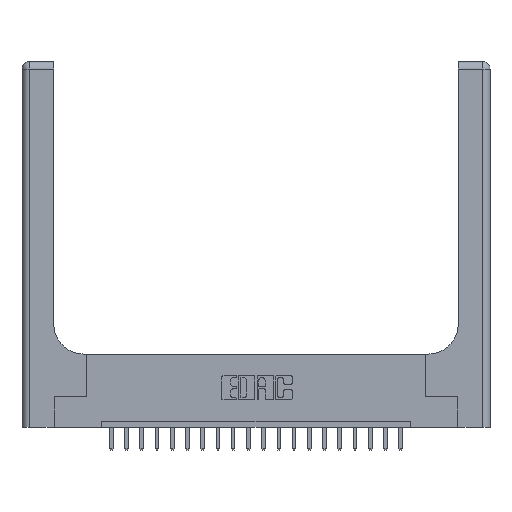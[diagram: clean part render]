
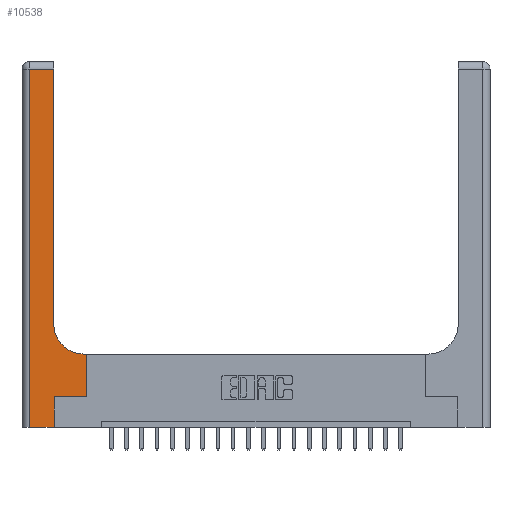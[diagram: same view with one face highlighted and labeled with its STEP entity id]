
A CAD part, top view. The second image highlights one B-rep face of the part: STEP entity #10538.
In plain terms, the highlighted planar face has unit normal (0, 0, 1).
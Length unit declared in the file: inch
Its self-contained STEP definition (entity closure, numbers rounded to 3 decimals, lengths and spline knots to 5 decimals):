
#203 = DIRECTION ( 'NONE',  ( 0., -1., 0. ) ) ;
#1177 = DIRECTION ( 'NONE',  ( 1., 0., 0. ) ) ;
#1221 = VECTOR ( 'NONE', #18222, 39.37008 ) ;
#1349 = CARTESIAN_POINT ( 'NONE',  ( 0.265, 0.25, 0.37 ) ) ;
#1490 = DIRECTION ( 'NONE',  ( 0., 1., 0. ) ) ;
#1596 = DIRECTION ( 'NONE',  ( 0., 0., -1. ) ) ;
#1726 = VECTOR ( 'NONE', #203, 39.37008 ) ;
#2391 = EDGE_CURVE ( 'NONE', #17876, #12855, #10352, .T. ) ;
#2981 = CARTESIAN_POINT ( 'NONE',  ( 0.51, 0.85, 0.37 ) ) ;
#3082 = ORIENTED_EDGE ( 'NONE', *, *, #6459, .T. ) ;
#4168 = LINE ( 'NONE', #12697, #9142 ) ;
#4330 = CARTESIAN_POINT ( 'NONE',  ( 0.26, 0.85, 0.37 ) ) ;
#4961 = ORIENTED_EDGE ( 'NONE', *, *, #12936, .T. ) ;
#4981 = ORIENTED_EDGE ( 'NONE', *, *, #11294, .T. ) ;
#5397 = EDGE_CURVE ( 'NONE', #9587, #10948, #16227, .T. ) ;
#5666 = AXIS2_PLACEMENT_3D ( 'NONE', #2981, #1596, #11240 ) ;
#5792 = VECTOR ( 'NONE', #6919, 39.37008 ) ;
#6413 = VERTEX_POINT ( 'NONE', #15447 ) ;
#6459 = EDGE_CURVE ( 'NONE', #13026, #11621, #8412, .T. ) ;
#6919 = DIRECTION ( 'NONE',  ( -1., 0., 0. ) ) ;
#7053 = DIRECTION ( 'NONE',  ( 1., 0., 0. ) ) ;
#7265 = EDGE_CURVE ( 'NONE', #11621, #8614, #4168, .T. ) ;
#7586 = VERTEX_POINT ( 'NONE', #11899 ) ;
#7779 = CARTESIAN_POINT ( 'NONE',  ( 0.06, 2.94, 0.37 ) ) ;
#8412 = LINE ( 'NONE', #17156, #13723 ) ;
#8614 = VERTEX_POINT ( 'NONE', #20523 ) ;
#8713 = LINE ( 'NONE', #10435, #1221 ) ;
#8873 = CARTESIAN_POINT ( 'NONE',  ( 0., 3., 0.37 ) ) ;
#8948 = DIRECTION ( 'NONE',  ( -1., 0., 0. ) ) ;
#8964 = DIRECTION ( 'NONE',  ( 0., 1., 0. ) ) ;
#9091 = EDGE_CURVE ( 'NONE', #8614, #17876, #10080, .T. ) ;
#9117 = ORIENTED_EDGE ( 'NONE', *, *, #2391, .T. ) ;
#9142 = VECTOR ( 'NONE', #8964, 39.37008 ) ;
#9587 = VERTEX_POINT ( 'NONE', #7779 ) ;
#9918 = ORIENTED_EDGE ( 'NONE', *, *, #7265, .T. ) ;
#10080 = LINE ( 'NONE', #14571, #5792 ) ;
#10352 = CIRCLE ( 'NONE', #5666, 0.25 ) ;
#10424 = VECTOR ( 'NONE', #7053, 39.37008 ) ;
#10435 = CARTESIAN_POINT ( 'NONE',  ( 0.26, 3., 0.37 ) ) ;
#10538 = ADVANCED_FACE ( 'NONE', ( #10584 ), #13402, .F. ) ;
#10584 = FACE_OUTER_BOUND ( 'NONE', #20178, .T. ) ;
#10661 = CARTESIAN_POINT ( 'NONE',  ( 0., 2.94, 0.37 ) ) ;
#10948 = VERTEX_POINT ( 'NONE', #11444 ) ;
#11061 = CARTESIAN_POINT ( 'NONE',  ( 0.265, 0., 0.37 ) ) ;
#11240 = DIRECTION ( 'NONE',  ( 1., 0., 0. ) ) ;
#11294 = EDGE_CURVE ( 'NONE', #6413, #9587, #17257, .T. ) ;
#11444 = CARTESIAN_POINT ( 'NONE',  ( 0.06, 0., 0.37 ) ) ;
#11621 = VERTEX_POINT ( 'NONE', #17534 ) ;
#11673 = ORIENTED_EDGE ( 'NONE', *, *, #13120, .T. ) ;
#11899 = CARTESIAN_POINT ( 'NONE',  ( 0.265, 0., 0.37 ) ) ;
#12366 = ORIENTED_EDGE ( 'NONE', *, *, #15570, .T. ) ;
#12381 = ORIENTED_EDGE ( 'NONE', *, *, #9091, .T. ) ;
#12697 = CARTESIAN_POINT ( 'NONE',  ( 0.528, 0.25, 0.37 ) ) ;
#12751 = VECTOR ( 'NONE', #1490, 39.37008 ) ;
#12855 = VERTEX_POINT ( 'NONE', #4330 ) ;
#12936 = EDGE_CURVE ( 'NONE', #7586, #13026, #13010, .T. ) ;
#13010 = LINE ( 'NONE', #11061, #12751 ) ;
#13026 = VERTEX_POINT ( 'NONE', #1349 ) ;
#13120 = EDGE_CURVE ( 'NONE', #12855, #6413, #8713, .T. ) ;
#13402 = PLANE ( 'NONE',  #19015 ) ;
#13723 = VECTOR ( 'NONE', #1177, 39.37008 ) ;
#14036 = ORIENTED_EDGE ( 'NONE', *, *, #5397, .T. ) ;
#14571 = CARTESIAN_POINT ( 'NONE',  ( 0.26, 0.6, 0.37 ) ) ;
#14699 = LINE ( 'NONE', #16527, #10424 ) ;
#14955 = CARTESIAN_POINT ( 'NONE',  ( 0.51, 0.6, 0.37 ) ) ;
#15447 = CARTESIAN_POINT ( 'NONE',  ( 0.26, 2.94, 0.37 ) ) ;
#15488 = DIRECTION ( 'NONE',  ( -1., 0., 0. ) ) ;
#15570 = EDGE_CURVE ( 'NONE', #10948, #7586, #14699, .T. ) ;
#16227 = LINE ( 'NONE', #19388, #1726 ) ;
#16527 = CARTESIAN_POINT ( 'NONE',  ( 0., 0., 0.37 ) ) ;
#16786 = VECTOR ( 'NONE', #15488, 39.37008 ) ;
#16836 = DIRECTION ( 'NONE',  ( 0., 0., -1. ) ) ;
#17156 = CARTESIAN_POINT ( 'NONE',  ( 0.265, 0.25, 0.37 ) ) ;
#17257 = LINE ( 'NONE', #10661, #16786 ) ;
#17534 = CARTESIAN_POINT ( 'NONE',  ( 0.528, 0.25, 0.37 ) ) ;
#17876 = VERTEX_POINT ( 'NONE', #14955 ) ;
#18222 = DIRECTION ( 'NONE',  ( 0., 1., 0. ) ) ;
#19015 = AXIS2_PLACEMENT_3D ( 'NONE', #8873, #16836, #8948 ) ;
#19388 = CARTESIAN_POINT ( 'NONE',  ( 0.06, 3., 0.37 ) ) ;
#20178 = EDGE_LOOP ( 'NONE', ( #11673, #4981, #14036, #12366, #4961, #3082, #9918, #12381, #9117 ) ) ;
#20523 = CARTESIAN_POINT ( 'NONE',  ( 0.528, 0.6, 0.37 ) ) ;
